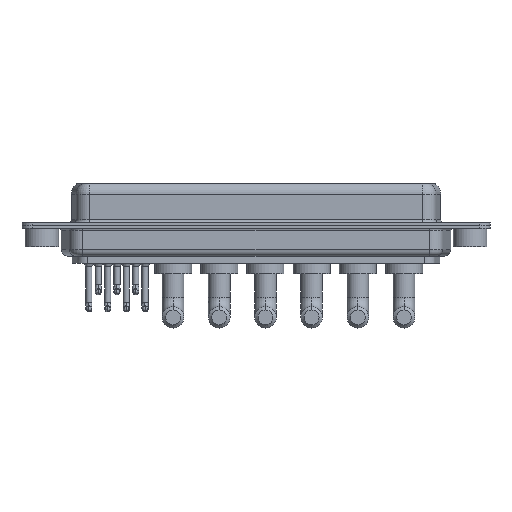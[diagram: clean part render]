
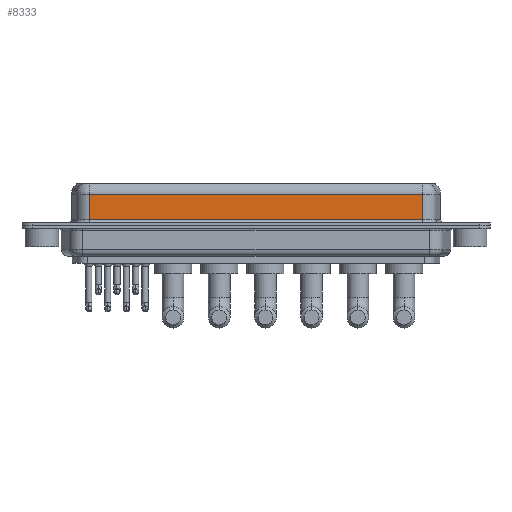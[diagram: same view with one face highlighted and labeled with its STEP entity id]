
A CAD part, front view. The second image highlights one B-rep face of the part: STEP entity #8333.
In plain terms, the highlighted planar face has unit normal (0, -1, 0).
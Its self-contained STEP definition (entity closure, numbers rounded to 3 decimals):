
#192 = DIRECTION ( 'NONE',  ( 1., 0., 0. ) ) ;
#295 = LINE ( 'NONE', #7630, #16716 ) ;
#1240 = AXIS2_PLACEMENT_3D ( 'NONE', #3232, #11722, #8781 ) ;
#1807 = CARTESIAN_POINT ( 'NONE',  ( 7.038, -3.95, 6.4 ) ) ;
#2822 = DIRECTION ( 'NONE',  ( -1., 0., 0. ) ) ;
#3124 = DIRECTION ( 'NONE',  ( 0., 0., -1. ) ) ;
#3232 = CARTESIAN_POINT ( 'NONE',  ( 56.462, -3.95, 6.4 ) ) ;
#3278 = VERTEX_POINT ( 'NONE', #17739 ) ;
#3395 = EDGE_CURVE ( 'NONE', #17075, #10447, #7263, .T. ) ;
#4187 = EDGE_LOOP ( 'NONE', ( #6313, #4890, #4470, #13872 ) ) ;
#4253 = VECTOR ( 'NONE', #3124, 1000. ) ;
#4445 = EDGE_CURVE ( 'NONE', #4634, #10447, #295, .T. ) ;
#4470 = ORIENTED_EDGE ( 'NONE', *, *, #17285, .T. ) ;
#4634 = VERTEX_POINT ( 'NONE', #13648 ) ;
#4890 = ORIENTED_EDGE ( 'NONE', *, *, #12926, .T. ) ;
#5714 = VECTOR ( 'NONE', #2822, 1000. ) ;
#6086 = LINE ( 'NONE', #1807, #4253 ) ;
#6313 = ORIENTED_EDGE ( 'NONE', *, *, #4445, .F. ) ;
#6900 = LINE ( 'NONE', #11331, #5714 ) ;
#7263 = LINE ( 'NONE', #12022, #8636 ) ;
#7630 = CARTESIAN_POINT ( 'NONE',  ( 56.462, -3.95, 6.4 ) ) ;
#7723 = DIRECTION ( 'NONE',  ( 0., 0., -1. ) ) ;
#8333 = ADVANCED_FACE ( 'NONE', ( #10187 ), #15876, .F. ) ;
#8636 = VECTOR ( 'NONE', #192, 1000. ) ;
#8781 = DIRECTION ( 'NONE',  ( 0., 0., 1. ) ) ;
#10187 = FACE_OUTER_BOUND ( 'NONE', #4187, .T. ) ;
#10447 = VERTEX_POINT ( 'NONE', #13190 ) ;
#11331 = CARTESIAN_POINT ( 'NONE',  ( 56.462, -3.95, 4.65 ) ) ;
#11722 = DIRECTION ( 'NONE',  ( 0., 1., 0. ) ) ;
#12022 = CARTESIAN_POINT ( 'NONE',  ( 56.462, -3.95, 0.9 ) ) ;
#12926 = EDGE_CURVE ( 'NONE', #4634, #3278, #6900, .T. ) ;
#13190 = CARTESIAN_POINT ( 'NONE',  ( 56.462, -3.95, 0.9 ) ) ;
#13540 = CARTESIAN_POINT ( 'NONE',  ( 7.038, -3.95, 0.9 ) ) ;
#13648 = CARTESIAN_POINT ( 'NONE',  ( 56.462, -3.95, 4.65 ) ) ;
#13872 = ORIENTED_EDGE ( 'NONE', *, *, #3395, .T. ) ;
#15876 = PLANE ( 'NONE',  #1240 ) ;
#16716 = VECTOR ( 'NONE', #7723, 1000. ) ;
#17075 = VERTEX_POINT ( 'NONE', #13540 ) ;
#17285 = EDGE_CURVE ( 'NONE', #3278, #17075, #6086, .T. ) ;
#17739 = CARTESIAN_POINT ( 'NONE',  ( 7.038, -3.95, 4.65 ) ) ;
